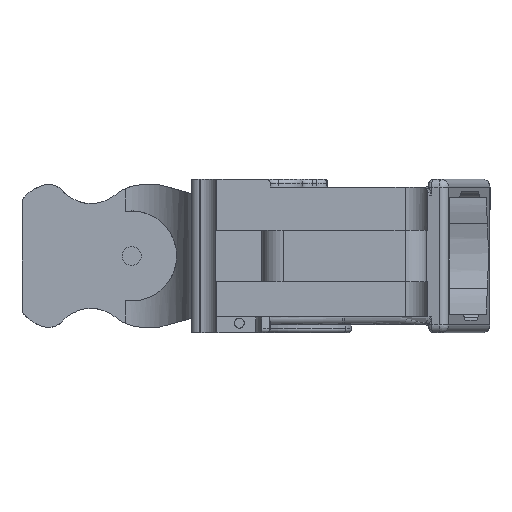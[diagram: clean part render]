
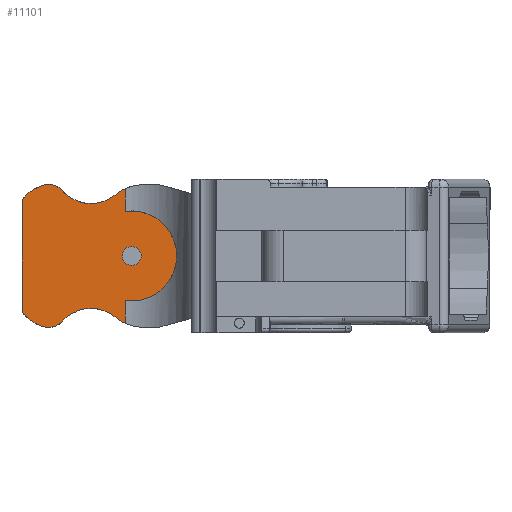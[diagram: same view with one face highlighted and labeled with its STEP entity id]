
A CAD part, left-side view. The second image highlights one B-rep face of the part: STEP entity #11101.
In plain terms, the highlighted planar face has unit normal (-1, 0, 0).
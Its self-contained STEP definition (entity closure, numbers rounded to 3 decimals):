
#240=FACE_BOUND('',#1703,.T.);
#1023=FACE_OUTER_BOUND('',#1702,.T.);
#1702=EDGE_LOOP('',(#8323,#8324,#8325,#8326,#8327,#8328,#8329,#8330,#8331,
#8332,#8333,#8334));
#1703=EDGE_LOOP('',(#8335));
#2438=CIRCLE('',#12008,11.25);
#2439=CIRCLE('',#12010,11.71);
#2440=CIRCLE('',#12011,9.539);
#2441=CIRCLE('',#12012,4.755);
#2442=CIRCLE('',#12013,9.022);
#2443=CIRCLE('',#12014,9.022);
#2444=CIRCLE('',#12015,4.755);
#2445=CIRCLE('',#12016,9.539);
#2446=CIRCLE('',#12017,11.71);
#2447=CIRCLE('',#12018,2.375);
#3159=LINE('',#22633,#3945);
#3162=LINE('',#22688,#3948);
#3163=LINE('',#22704,#3949);
#3945=VECTOR('',#14011,10.);
#3948=VECTOR('',#14024,10.);
#3949=VECTOR('',#14041,10.);
#4934=VERTEX_POINT('',#22630);
#4935=VERTEX_POINT('',#22632);
#4938=VERTEX_POINT('',#22653);
#4939=VERTEX_POINT('',#22654);
#4940=VERTEX_POINT('',#22687);
#4941=VERTEX_POINT('',#22689);
#4942=VERTEX_POINT('',#22691);
#4943=VERTEX_POINT('',#22693);
#4944=VERTEX_POINT('',#22696);
#4945=VERTEX_POINT('',#22698);
#4946=VERTEX_POINT('',#22700);
#4947=VERTEX_POINT('',#22702);
#4948=VERTEX_POINT('',#22705);
#6195=EDGE_CURVE('',#4935,#4934,#3159,.F.);
#6201=EDGE_CURVE('',#4939,#4938,#2438,.T.);
#6202=EDGE_CURVE('',#4940,#4938,#3162,.T.);
#6203=EDGE_CURVE('',#4940,#4941,#2439,.F.);
#6204=EDGE_CURVE('',#4941,#4942,#2440,.F.);
#6205=EDGE_CURVE('',#4942,#4943,#2441,.F.);
#6206=EDGE_CURVE('',#4943,#4935,#2442,.F.);
#6207=EDGE_CURVE('',#4934,#4944,#2443,.F.);
#6208=EDGE_CURVE('',#4944,#4945,#2444,.F.);
#6209=EDGE_CURVE('',#4945,#4946,#2445,.F.);
#6210=EDGE_CURVE('',#4946,#4947,#2446,.F.);
#6211=EDGE_CURVE('',#4939,#4947,#3163,.T.);
#6212=EDGE_CURVE('',#4948,#4948,#2447,.T.);
#8323=ORIENTED_EDGE('',*,*,#6201,.T.);
#8324=ORIENTED_EDGE('',*,*,#6202,.F.);
#8325=ORIENTED_EDGE('',*,*,#6203,.T.);
#8326=ORIENTED_EDGE('',*,*,#6204,.T.);
#8327=ORIENTED_EDGE('',*,*,#6205,.T.);
#8328=ORIENTED_EDGE('',*,*,#6206,.T.);
#8329=ORIENTED_EDGE('',*,*,#6195,.T.);
#8330=ORIENTED_EDGE('',*,*,#6207,.T.);
#8331=ORIENTED_EDGE('',*,*,#6208,.T.);
#8332=ORIENTED_EDGE('',*,*,#6209,.T.);
#8333=ORIENTED_EDGE('',*,*,#6210,.T.);
#8334=ORIENTED_EDGE('',*,*,#6211,.F.);
#8335=ORIENTED_EDGE('',*,*,#6212,.F.);
#10782=PLANE('',#12009);
#11101=ADVANCED_FACE('',(#1023,#240),#10782,.T.);
#12008=AXIS2_PLACEMENT_3D('',#22685,#14020,#14021);
#12009=AXIS2_PLACEMENT_3D('',#22686,#14022,#14023);
#12010=AXIS2_PLACEMENT_3D('',#22690,#14025,#14026);
#12011=AXIS2_PLACEMENT_3D('',#22692,#14027,#14028);
#12012=AXIS2_PLACEMENT_3D('',#22694,#14029,#14030);
#12013=AXIS2_PLACEMENT_3D('',#22695,#14031,#14032);
#12014=AXIS2_PLACEMENT_3D('',#22697,#14033,#14034);
#12015=AXIS2_PLACEMENT_3D('',#22699,#14035,#14036);
#12016=AXIS2_PLACEMENT_3D('',#22701,#14037,#14038);
#12017=AXIS2_PLACEMENT_3D('',#22703,#14039,#14040);
#12018=AXIS2_PLACEMENT_3D('',#22706,#14042,#14043);
#14011=DIRECTION('',(0.,0.,1.));
#14020=DIRECTION('center_axis',(-1.,0.,0.));
#14021=DIRECTION('ref_axis',(0.,-1.,0.));
#14022=DIRECTION('center_axis',(-1.,0.,0.));
#14023=DIRECTION('ref_axis',(0.,-1.,0.));
#14024=DIRECTION('',(0.,0.,-1.));
#14025=DIRECTION('center_axis',(1.,0.,0.));
#14026=DIRECTION('ref_axis',(0.,1.,0.));
#14027=DIRECTION('center_axis',(-1.,0.,0.));
#14028=DIRECTION('ref_axis',(0.,1.,0.));
#14029=DIRECTION('center_axis',(1.,0.,0.));
#14030=DIRECTION('ref_axis',(0.,1.,0.));
#14031=DIRECTION('center_axis',(1.,0.,0.));
#14032=DIRECTION('ref_axis',(0.,1.,0.));
#14033=DIRECTION('center_axis',(1.,0.,0.));
#14034=DIRECTION('ref_axis',(0.,1.,0.));
#14035=DIRECTION('center_axis',(1.,0.,0.));
#14036=DIRECTION('ref_axis',(0.,1.,0.));
#14037=DIRECTION('center_axis',(-1.,0.,0.));
#14038=DIRECTION('ref_axis',(0.,1.,0.));
#14039=DIRECTION('center_axis',(1.,0.,0.));
#14040=DIRECTION('ref_axis',(0.,1.,0.));
#14041=DIRECTION('',(0.,0.,-1.));
#14042=DIRECTION('center_axis',(-1.,0.,0.));
#14043=DIRECTION('ref_axis',(0.,-1.,0.));
#22630=CARTESIAN_POINT('',(593.557,210.383,-0.109));
#22632=CARTESIAN_POINT('',(593.557,210.383,27.568));
#22633=CARTESIAN_POINT('',(593.557,210.383,13.73));
#22653=CARTESIAN_POINT('',(593.557,184.533,24.869));
#22654=CARTESIAN_POINT('',(593.557,184.533,2.59));
#22685=CARTESIAN_POINT('Origin',(593.557,182.958,13.73));
#22686=CARTESIAN_POINT('Origin',(593.557,211.383,13.73));
#22687=CARTESIAN_POINT('',(593.557,184.533,30.555));
#22688=CARTESIAN_POINT('',(593.557,184.533,5.021));
#22689=CARTESIAN_POINT('',(593.557,187.122,28.962));
#22690=CARTESIAN_POINT('Origin',(593.557,179.743,19.87));
#22691=CARTESIAN_POINT('',(593.557,200.235,29.999));
#22692=CARTESIAN_POINT('Origin',(593.557,193.133,36.369));
#22693=CARTESIAN_POINT('',(593.557,205.765,31.143));
#22694=CARTESIAN_POINT('Origin',(593.557,203.774,26.824));
#22695=CARTESIAN_POINT('Origin',(593.557,202.849,22.606));
#22696=CARTESIAN_POINT('',(593.557,205.765,-3.684));
#22697=CARTESIAN_POINT('Origin',(593.557,202.849,4.854));
#22698=CARTESIAN_POINT('',(593.557,200.235,-2.54));
#22699=CARTESIAN_POINT('Origin',(593.557,203.774,0.635));
#22700=CARTESIAN_POINT('',(593.557,187.122,-1.503));
#22701=CARTESIAN_POINT('Origin',(593.557,193.133,-8.91));
#22702=CARTESIAN_POINT('',(593.557,184.533,-3.096));
#22703=CARTESIAN_POINT('Origin',(593.557,179.743,7.589));
#22704=CARTESIAN_POINT('',(593.557,184.533,5.021));
#22705=CARTESIAN_POINT('',(593.557,185.333,13.73));
#22706=CARTESIAN_POINT('Origin',(593.557,182.958,13.73));
